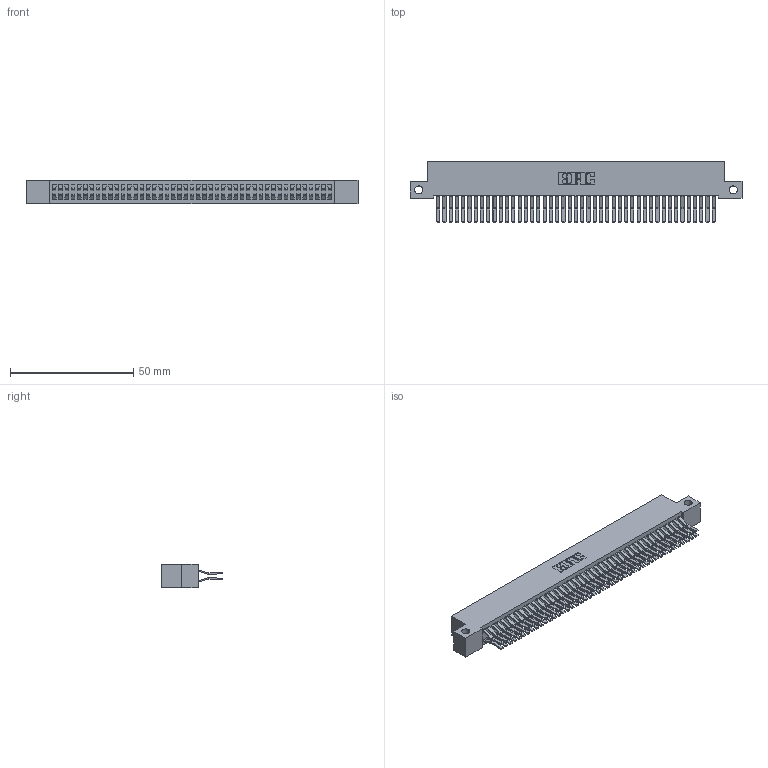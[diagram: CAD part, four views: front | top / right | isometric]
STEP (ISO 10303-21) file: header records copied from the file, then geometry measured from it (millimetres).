
FILE_DESCRIPTION (( 'STEP AP203' ), '1' );
FILE_NAME ('342-090-560-212.STEP', '2018-08-14T01:31:25', ( '' ), ( '' ), 'SwSTEP 2.0', 'SolidWorks 2016', '' );
FILE_SCHEMA (( 'CONFIG_CONTROL_DESIGN' ));
Length unit declared in the file: inch
Products named in the file (3): 345-292-001_560 Tail; 342-090-560-212; 342 Part_Side Mount
Assembly tree (91 placements, depth 2):
  342-090-560-212
    342 Part_Side Mount
    345-292-001_560 Tail  x90
Bounding box: 134.62 x 24.78 x 9.4 mm (x, y, z)
Volume: 12626.7 mm3; surface area: 21884.2 mm2
Topology: 91 solids, 91 shells, 4970 faces, 14789 edges, 9738 vertices
Faces by surface type: plane 3306, cylinder 1664
Entity records: 28521 total; most frequent: CARTESIAN_POINT 4722, ORIENTED_EDGE 4658, DIRECTION 4033, EDGE_CURVE 2329, LINE 2197, VECTOR 2197, VERTEX_POINT 1550, AXIS2_PLACEMENT_3D 918
